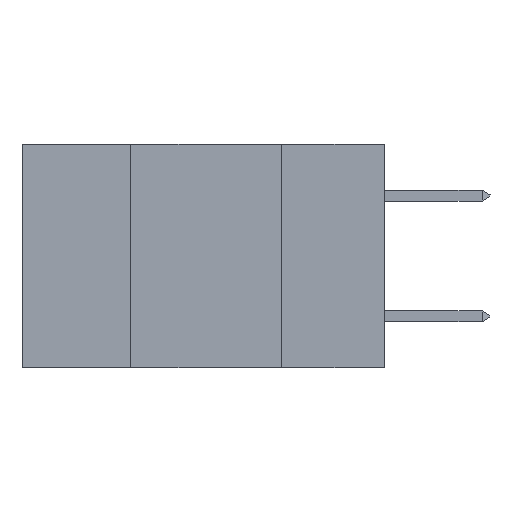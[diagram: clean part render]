
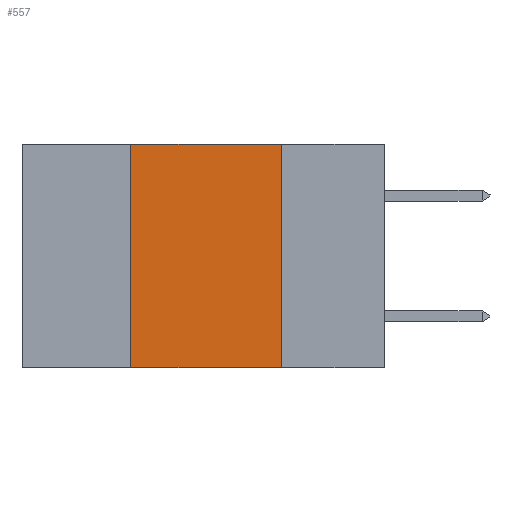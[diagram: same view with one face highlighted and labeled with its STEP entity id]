
A CAD part, left-side view. The second image highlights one B-rep face of the part: STEP entity #557.
In plain terms, the highlighted planar face has unit normal (-1, 0, 0).
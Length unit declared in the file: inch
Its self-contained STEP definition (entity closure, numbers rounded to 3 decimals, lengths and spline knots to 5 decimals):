
#557 = ADVANCED_FACE ( 'NONE', ( #16899 ), #21700, .F. ) ;
#911 = EDGE_CURVE ( 'NONE', #26237, #15461, #27959, .T. ) ;
#2237 = AXIS2_PLACEMENT_3D ( 'NONE', #21943, #4474, #36153 ) ;
#4474 = DIRECTION ( 'NONE',  ( 1., 0., 0. ) ) ;
#5467 = LINE ( 'NONE', #8344, #27887 ) ;
#6048 = CARTESIAN_POINT ( 'NONE',  ( 0., 0.6, -0.37 ) ) ;
#7310 = VERTEX_POINT ( 'NONE', #37169 ) ;
#7323 = ORIENTED_EDGE ( 'NONE', *, *, #32925, .F. ) ;
#7717 = LINE ( 'NONE', #6048, #33818 ) ;
#8344 = CARTESIAN_POINT ( 'NONE',  ( 0., 0.17, 0. ) ) ;
#9709 = VERTEX_POINT ( 'NONE', #31323 ) ;
#10094 = VECTOR ( 'NONE', #23686, 39.37008 ) ;
#10681 = ORIENTED_EDGE ( 'NONE', *, *, #19272, .T. ) ;
#12412 = EDGE_CURVE ( 'NONE', #15461, #7310, #5467, .T. ) ;
#12577 = LINE ( 'NONE', #15241, #25396 ) ;
#15241 = CARTESIAN_POINT ( 'NONE',  ( 0., 0.42, 0. ) ) ;
#15461 = VERTEX_POINT ( 'NONE', #26142 ) ;
#16899 = FACE_OUTER_BOUND ( 'NONE', #34888, .T. ) ;
#19272 = EDGE_CURVE ( 'NONE', #9709, #7310, #7717, .T. ) ;
#20717 = CARTESIAN_POINT ( 'NONE',  ( 0., 0.6, 0. ) ) ;
#21700 = PLANE ( 'NONE',  #2237 ) ;
#21943 = CARTESIAN_POINT ( 'NONE',  ( 0., 0.6, 0. ) ) ;
#23077 = DIRECTION ( 'NONE',  ( 0., -1., 0. ) ) ;
#23686 = DIRECTION ( 'NONE',  ( 0., -1., 0. ) ) ;
#24448 = ORIENTED_EDGE ( 'NONE', *, *, #12412, .F. ) ;
#25396 = VECTOR ( 'NONE', #35573, 39.37008 ) ;
#26142 = CARTESIAN_POINT ( 'NONE',  ( 0., 0.17, 0. ) ) ;
#26237 = VERTEX_POINT ( 'NONE', #34833 ) ;
#27663 = ORIENTED_EDGE ( 'NONE', *, *, #911, .F. ) ;
#27887 = VECTOR ( 'NONE', #35058, 39.37008 ) ;
#27959 = LINE ( 'NONE', #20717, #10094 ) ;
#31323 = CARTESIAN_POINT ( 'NONE',  ( 0., 0.42, -0.37 ) ) ;
#32925 = EDGE_CURVE ( 'NONE', #9709, #26237, #12577, .T. ) ;
#33818 = VECTOR ( 'NONE', #23077, 39.37008 ) ;
#34833 = CARTESIAN_POINT ( 'NONE',  ( 0., 0.42, 0. ) ) ;
#34888 = EDGE_LOOP ( 'NONE', ( #24448, #27663, #7323, #10681 ) ) ;
#35058 = DIRECTION ( 'NONE',  ( 0., 0., -1. ) ) ;
#35573 = DIRECTION ( 'NONE',  ( 0., 0., 1. ) ) ;
#36153 = DIRECTION ( 'NONE',  ( 0., 0., -1. ) ) ;
#37169 = CARTESIAN_POINT ( 'NONE',  ( 0., 0.17, -0.37 ) ) ;
